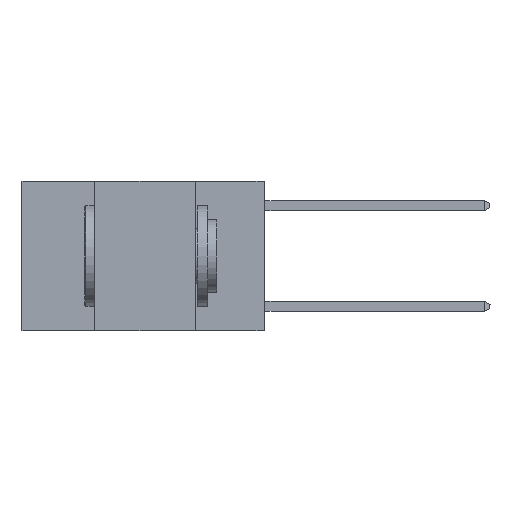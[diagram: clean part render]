
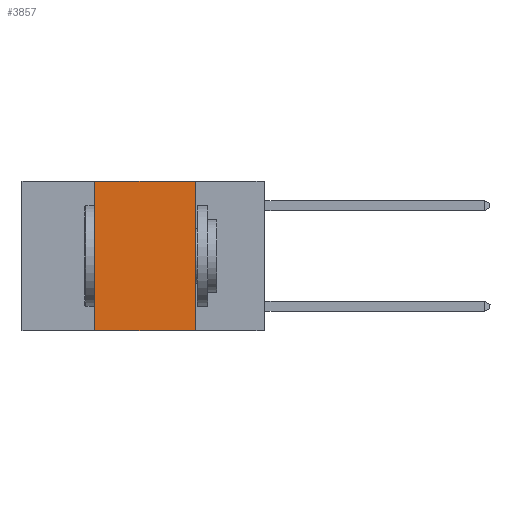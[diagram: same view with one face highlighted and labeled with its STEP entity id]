
A CAD part, left-side view. The second image highlights one B-rep face of the part: STEP entity #3857.
In plain terms, the highlighted planar face has unit normal (-1, 0, 0).
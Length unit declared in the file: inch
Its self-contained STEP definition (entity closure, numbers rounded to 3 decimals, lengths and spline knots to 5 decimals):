
#265 = DIRECTION ( 'NONE',  ( 0., -1., 0. ) ) ;
#281 = VECTOR ( 'NONE', #11180, 39.37008 ) ;
#823 = ORIENTED_EDGE ( 'NONE', *, *, #3819, .F. ) ;
#983 = CARTESIAN_POINT ( 'NONE',  ( 0., 0.42, 0. ) ) ;
#2726 = FACE_OUTER_BOUND ( 'NONE', #3966, .T. ) ;
#3334 = VERTEX_POINT ( 'NONE', #4643 ) ;
#3819 = EDGE_CURVE ( 'NONE', #12630, #3334, #7301, .T. ) ;
#3857 = ADVANCED_FACE ( 'NONE', ( #2726 ), #10194, .F. ) ;
#3966 = EDGE_LOOP ( 'NONE', ( #823, #12472, #8364, #12984 ) ) ;
#4471 = DIRECTION ( 'NONE',  ( 0., 0., -1. ) ) ;
#4643 = CARTESIAN_POINT ( 'NONE',  ( 0., 0.17, -0.37 ) ) ;
#6247 = LINE ( 'NONE', #13939, #12558 ) ;
#6658 = CARTESIAN_POINT ( 'NONE',  ( 0., 0.42, -0.37 ) ) ;
#7301 = LINE ( 'NONE', #12273, #281 ) ;
#7839 = CARTESIAN_POINT ( 'NONE',  ( 0., 0.17, 0. ) ) ;
#8054 = VERTEX_POINT ( 'NONE', #6658 ) ;
#8364 = ORIENTED_EDGE ( 'NONE', *, *, #14627, .F. ) ;
#8542 = VECTOR ( 'NONE', #10802, 39.37008 ) ;
#9119 = AXIS2_PLACEMENT_3D ( 'NONE', #13403, #11275, #4471 ) ;
#9270 = CARTESIAN_POINT ( 'NONE',  ( 0., 0.6, 0. ) ) ;
#10194 = PLANE ( 'NONE',  #9119 ) ;
#10397 = DIRECTION ( 'NONE',  ( 0., -1., 0. ) ) ;
#10802 = DIRECTION ( 'NONE',  ( 0., 0., 1. ) ) ;
#11034 = EDGE_CURVE ( 'NONE', #11839, #12630, #14621, .T. ) ;
#11180 = DIRECTION ( 'NONE',  ( 0., 0., -1. ) ) ;
#11275 = DIRECTION ( 'NONE',  ( 1., 0., 0. ) ) ;
#11495 = LINE ( 'NONE', #14067, #8542 ) ;
#11839 = VERTEX_POINT ( 'NONE', #983 ) ;
#12273 = CARTESIAN_POINT ( 'NONE',  ( 0., 0.17, 0. ) ) ;
#12472 = ORIENTED_EDGE ( 'NONE', *, *, #11034, .F. ) ;
#12558 = VECTOR ( 'NONE', #265, 39.37008 ) ;
#12630 = VERTEX_POINT ( 'NONE', #7839 ) ;
#12984 = ORIENTED_EDGE ( 'NONE', *, *, #13158, .T. ) ;
#13158 = EDGE_CURVE ( 'NONE', #8054, #3334, #6247, .T. ) ;
#13403 = CARTESIAN_POINT ( 'NONE',  ( 0., 0.6, 0. ) ) ;
#13939 = CARTESIAN_POINT ( 'NONE',  ( 0., 0.6, -0.37 ) ) ;
#14067 = CARTESIAN_POINT ( 'NONE',  ( 0., 0.42, 0. ) ) ;
#14275 = VECTOR ( 'NONE', #10397, 39.37008 ) ;
#14621 = LINE ( 'NONE', #9270, #14275 ) ;
#14627 = EDGE_CURVE ( 'NONE', #8054, #11839, #11495, .T. ) ;
